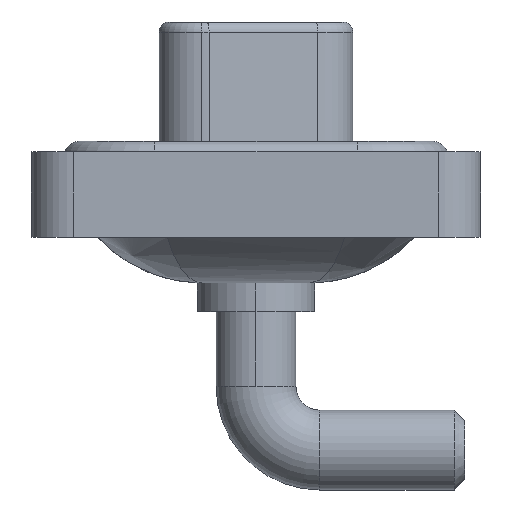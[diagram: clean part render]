
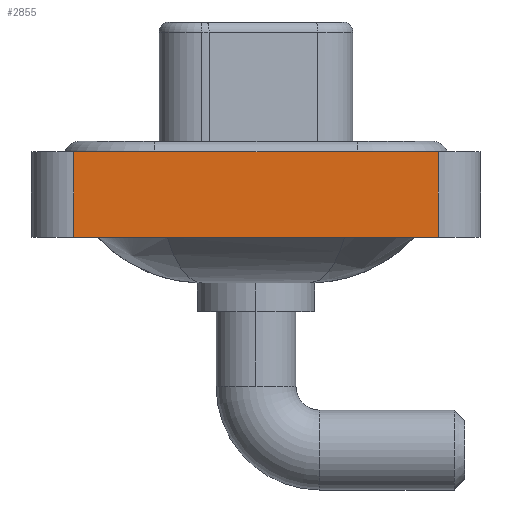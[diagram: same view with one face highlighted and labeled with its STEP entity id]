
A CAD part, left-side view. The second image highlights one B-rep face of the part: STEP entity #2855.
In plain terms, the highlighted planar face has unit normal (-1, 0, 0).
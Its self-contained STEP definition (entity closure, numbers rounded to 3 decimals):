
#246 = VECTOR ( 'NONE', #10036, 1000. ) ;
#718 = CARTESIAN_POINT ( 'NONE',  ( -7.3, -8.55, 0.4 ) ) ;
#1029 = LINE ( 'NONE', #4957, #246 ) ;
#1719 = CARTESIAN_POINT ( 'NONE',  ( -7.3, -8.55, -3.6 ) ) ;
#1913 = ORIENTED_EDGE ( 'NONE', *, *, #8313, .F. ) ;
#2697 = VERTEX_POINT ( 'NONE', #10238 ) ;
#2702 = DIRECTION ( 'NONE',  ( 0., 0., 1. ) ) ;
#2855 = ADVANCED_FACE ( 'NONE', ( #13127 ), #10637, .T. ) ;
#3089 = EDGE_CURVE ( 'NONE', #5168, #2697, #3634, .T. ) ;
#3634 = LINE ( 'NONE', #10050, #16427 ) ;
#3795 = CARTESIAN_POINT ( 'NONE',  ( -7.3, 8.55, -3.6 ) ) ;
#3859 = VERTEX_POINT ( 'NONE', #9608 ) ;
#4470 = DIRECTION ( 'NONE',  ( 0., 0., 1. ) ) ;
#4639 = CARTESIAN_POINT ( 'NONE',  ( -7.3, -8.55, -3.6 ) ) ;
#4890 = LINE ( 'NONE', #4639, #5905 ) ;
#4957 = CARTESIAN_POINT ( 'NONE',  ( -7.3, -8.55, 0.4 ) ) ;
#5168 = VERTEX_POINT ( 'NONE', #9688 ) ;
#5905 = VECTOR ( 'NONE', #9967, 1000. ) ;
#7137 = DIRECTION ( 'NONE',  ( -1., 0., 0. ) ) ;
#7714 = LINE ( 'NONE', #3795, #11679 ) ;
#8313 = EDGE_CURVE ( 'NONE', #5168, #3859, #7714, .T. ) ;
#8408 = EDGE_CURVE ( 'NONE', #3859, #16057, #1029, .T. ) ;
#9324 = ORIENTED_EDGE ( 'NONE', *, *, #3089, .T. ) ;
#9608 = CARTESIAN_POINT ( 'NONE',  ( -7.3, 8.55, 0.4 ) ) ;
#9688 = CARTESIAN_POINT ( 'NONE',  ( -7.3, 8.55, -3.6 ) ) ;
#9967 = DIRECTION ( 'NONE',  ( 0., 0., 1. ) ) ;
#10036 = DIRECTION ( 'NONE',  ( 0., -1., 0. ) ) ;
#10050 = CARTESIAN_POINT ( 'NONE',  ( -7.3, -8.55, -3.6 ) ) ;
#10238 = CARTESIAN_POINT ( 'NONE',  ( -7.3, -8.55, -3.6 ) ) ;
#10637 = PLANE ( 'NONE',  #15670 ) ;
#11679 = VECTOR ( 'NONE', #2702, 1000. ) ;
#12285 = DIRECTION ( 'NONE',  ( 0., -1., 0. ) ) ;
#13127 = FACE_OUTER_BOUND ( 'NONE', #15169, .T. ) ;
#13462 = EDGE_CURVE ( 'NONE', #2697, #16057, #4890, .T. ) ;
#14934 = ORIENTED_EDGE ( 'NONE', *, *, #13462, .T. ) ;
#15169 = EDGE_LOOP ( 'NONE', ( #14934, #15958, #1913, #9324 ) ) ;
#15670 = AXIS2_PLACEMENT_3D ( 'NONE', #1719, #7137, #4470 ) ;
#15958 = ORIENTED_EDGE ( 'NONE', *, *, #8408, .F. ) ;
#16057 = VERTEX_POINT ( 'NONE', #718 ) ;
#16427 = VECTOR ( 'NONE', #12285, 1000. ) ;
